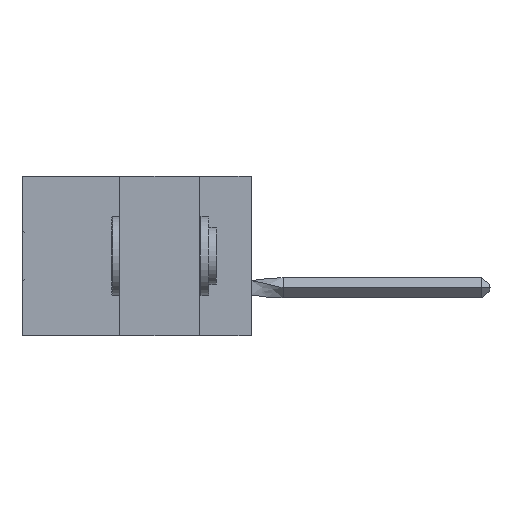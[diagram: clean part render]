
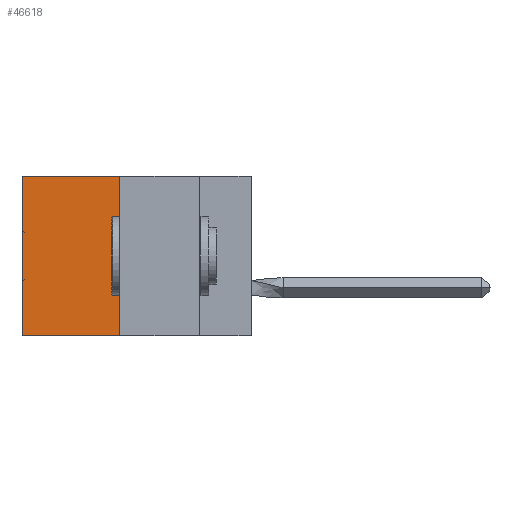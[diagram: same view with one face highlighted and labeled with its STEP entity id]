
A CAD part, left-side view. The second image highlights one B-rep face of the part: STEP entity #46618.
In plain terms, the highlighted planar face has unit normal (-1, 0, 0).
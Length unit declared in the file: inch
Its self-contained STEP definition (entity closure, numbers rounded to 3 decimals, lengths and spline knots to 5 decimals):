
#1036 = EDGE_LOOP ( 'NONE', ( #7178, #44186, #2505, #12190 ) ) ;
#1544 = PLANE ( 'NONE',  #4491 ) ;
#2505 = ORIENTED_EDGE ( 'NONE', *, *, #11639, .F. ) ;
#3026 = CARTESIAN_POINT ( 'NONE',  ( 0.305, 0.72, -0.5 ) ) ;
#4081 = LINE ( 'NONE', #26673, #11939 ) ;
#4491 = AXIS2_PLACEMENT_3D ( 'NONE', #20118, #16878, #36039 ) ;
#4578 = LINE ( 'NONE', #21919, #26931 ) ;
#7043 = CARTESIAN_POINT ( 'NONE',  ( 0.305, 0.413, -0.5 ) ) ;
#7178 = ORIENTED_EDGE ( 'NONE', *, *, #36251, .T. ) ;
#11639 = EDGE_CURVE ( 'NONE', #45287, #14222, #40259, .T. ) ;
#11939 = VECTOR ( 'NONE', #11962, 39.37008 ) ;
#11962 = DIRECTION ( 'NONE',  ( 0., 1., 0. ) ) ;
#12190 = ORIENTED_EDGE ( 'NONE', *, *, #18602, .T. ) ;
#13654 = DIRECTION ( 'NONE',  ( 0., 1., 0. ) ) ;
#13796 = VECTOR ( 'NONE', #39365, 39.37008 ) ;
#14222 = VERTEX_POINT ( 'NONE', #38806 ) ;
#14653 = EDGE_CURVE ( 'NONE', #14222, #20125, #4578, .T. ) ;
#16878 = DIRECTION ( 'NONE',  ( 1., 0., 0. ) ) ;
#18602 = EDGE_CURVE ( 'NONE', #45287, #46555, #4081, .T. ) ;
#20118 = CARTESIAN_POINT ( 'NONE',  ( 0.305, 0.413, -0.5 ) ) ;
#20125 = VERTEX_POINT ( 'NONE', #32564 ) ;
#21919 = CARTESIAN_POINT ( 'NONE',  ( 0.305, 0.413, -0.5 ) ) ;
#25446 = DIRECTION ( 'NONE',  ( 0., 0., -1. ) ) ;
#26673 = CARTESIAN_POINT ( 'NONE',  ( 0.305, 0.413, 0. ) ) ;
#26931 = VECTOR ( 'NONE', #13654, 39.37008 ) ;
#30606 = FACE_OUTER_BOUND ( 'NONE', #1036, .T. ) ;
#32564 = CARTESIAN_POINT ( 'NONE',  ( 0.305, 0.72, -0.5 ) ) ;
#35538 = CARTESIAN_POINT ( 'NONE',  ( 0.305, 0.72, 0. ) ) ;
#36039 = DIRECTION ( 'NONE',  ( 0., 0., -1. ) ) ;
#36251 = EDGE_CURVE ( 'NONE', #46555, #20125, #36832, .T. ) ;
#36832 = LINE ( 'NONE', #3026, #13796 ) ;
#38806 = CARTESIAN_POINT ( 'NONE',  ( 0.305, 0.413, -0.5 ) ) ;
#39365 = DIRECTION ( 'NONE',  ( 0., 0., -1. ) ) ;
#39522 = CARTESIAN_POINT ( 'NONE',  ( 0.305, 0.413, 0. ) ) ;
#40259 = LINE ( 'NONE', #7043, #43278 ) ;
#43278 = VECTOR ( 'NONE', #25446, 39.37008 ) ;
#44186 = ORIENTED_EDGE ( 'NONE', *, *, #14653, .F. ) ;
#45287 = VERTEX_POINT ( 'NONE', #39522 ) ;
#46555 = VERTEX_POINT ( 'NONE', #35538 ) ;
#46618 = ADVANCED_FACE ( 'NONE', ( #30606 ), #1544, .F. ) ;
